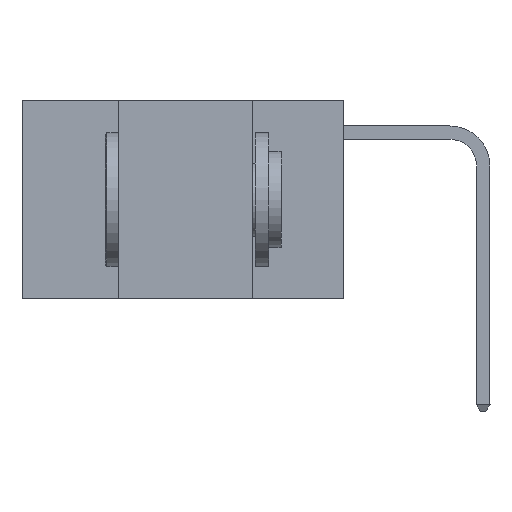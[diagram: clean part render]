
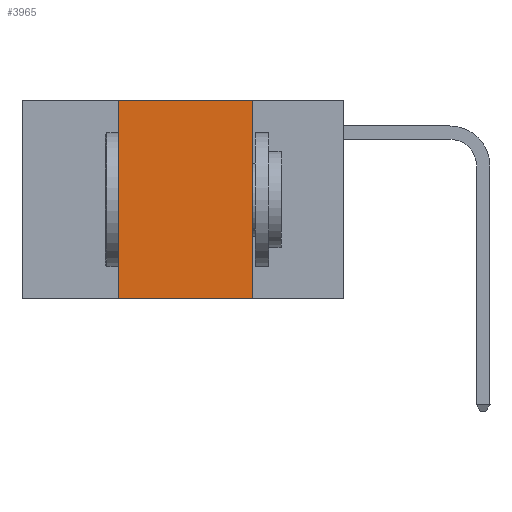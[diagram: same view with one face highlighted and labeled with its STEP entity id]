
A CAD part, left-side view. The second image highlights one B-rep face of the part: STEP entity #3965.
In plain terms, the highlighted planar face has unit normal (-1, 0, 0).
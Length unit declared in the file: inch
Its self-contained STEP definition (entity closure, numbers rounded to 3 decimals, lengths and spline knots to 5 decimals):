
#203 = ORIENTED_EDGE ( 'NONE', *, *, #4467, .T. ) ;
#209 = DIRECTION ( 'NONE',  ( 0., 0., -1. ) ) ;
#1144 = VERTEX_POINT ( 'NONE', #13163 ) ;
#3680 = AXIS2_PLACEMENT_3D ( 'NONE', #4545, #8864, #209 ) ;
#3965 = ADVANCED_FACE ( 'NONE', ( #5533 ), #17474, .F. ) ;
#4093 = CARTESIAN_POINT ( 'NONE',  ( 0., 0.17, 0. ) ) ;
#4464 = CARTESIAN_POINT ( 'NONE',  ( 0., 0.42, 0. ) ) ;
#4467 = EDGE_CURVE ( 'NONE', #14643, #1144, #7509, .T. ) ;
#4509 = ORIENTED_EDGE ( 'NONE', *, *, #12057, .F. ) ;
#4535 = ORIENTED_EDGE ( 'NONE', *, *, #16981, .F. ) ;
#4545 = CARTESIAN_POINT ( 'NONE',  ( 0., 0.6, 0. ) ) ;
#4556 = CARTESIAN_POINT ( 'NONE',  ( 0., 0.6, -0.37 ) ) ;
#4991 = VECTOR ( 'NONE', #11839, 39.37008 ) ;
#5533 = FACE_OUTER_BOUND ( 'NONE', #16920, .T. ) ;
#6023 = DIRECTION ( 'NONE',  ( 0., -1., 0. ) ) ;
#6053 = CARTESIAN_POINT ( 'NONE',  ( 0., 0.42, 0. ) ) ;
#6316 = LINE ( 'NONE', #7219, #13487 ) ;
#6566 = ORIENTED_EDGE ( 'NONE', *, *, #13957, .F. ) ;
#7219 = CARTESIAN_POINT ( 'NONE',  ( 0., 0.17, 0. ) ) ;
#7509 = LINE ( 'NONE', #4556, #14689 ) ;
#7760 = VERTEX_POINT ( 'NONE', #4093 ) ;
#8652 = DIRECTION ( 'NONE',  ( 0., 0., -1. ) ) ;
#8864 = DIRECTION ( 'NONE',  ( 1., 0., 0. ) ) ;
#9063 = CARTESIAN_POINT ( 'NONE',  ( 0., 0.42, -0.37 ) ) ;
#10281 = DIRECTION ( 'NONE',  ( 0., 0., 1. ) ) ;
#10297 = VECTOR ( 'NONE', #10281, 39.37008 ) ;
#10384 = CARTESIAN_POINT ( 'NONE',  ( 0., 0.6, 0. ) ) ;
#10849 = VERTEX_POINT ( 'NONE', #4464 ) ;
#11839 = DIRECTION ( 'NONE',  ( 0., -1., 0. ) ) ;
#12057 = EDGE_CURVE ( 'NONE', #10849, #7760, #15997, .T. ) ;
#13163 = CARTESIAN_POINT ( 'NONE',  ( 0., 0.17, -0.37 ) ) ;
#13487 = VECTOR ( 'NONE', #8652, 39.37008 ) ;
#13957 = EDGE_CURVE ( 'NONE', #7760, #1144, #6316, .T. ) ;
#14643 = VERTEX_POINT ( 'NONE', #9063 ) ;
#14689 = VECTOR ( 'NONE', #6023, 39.37008 ) ;
#15997 = LINE ( 'NONE', #10384, #4991 ) ;
#16920 = EDGE_LOOP ( 'NONE', ( #6566, #4509, #4535, #203 ) ) ;
#16981 = EDGE_CURVE ( 'NONE', #14643, #10849, #17954, .T. ) ;
#17474 = PLANE ( 'NONE',  #3680 ) ;
#17954 = LINE ( 'NONE', #6053, #10297 ) ;
